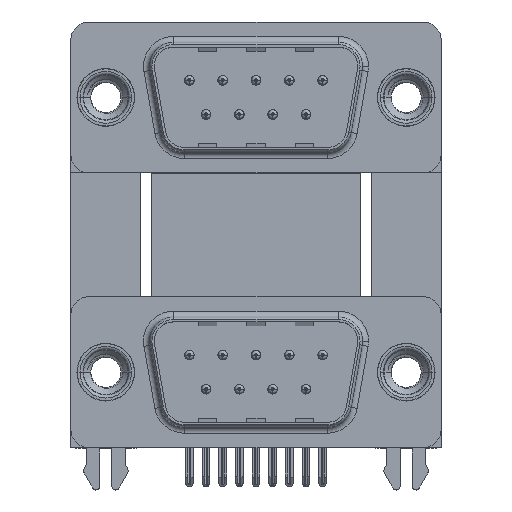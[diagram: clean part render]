
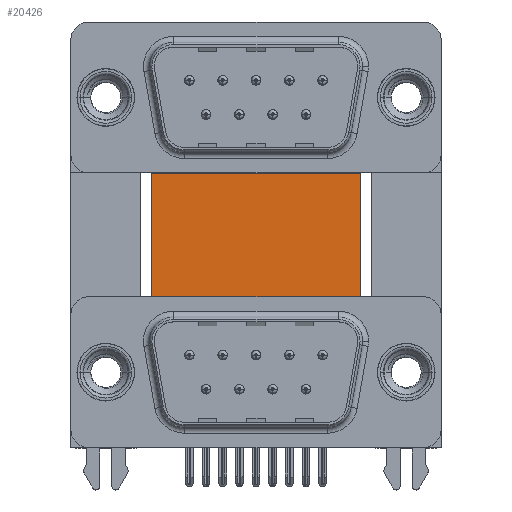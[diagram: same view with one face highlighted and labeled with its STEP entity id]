
A CAD part, top view. The second image highlights one B-rep face of the part: STEP entity #20426.
In plain terms, the highlighted planar face has unit normal (0, 0, 1).
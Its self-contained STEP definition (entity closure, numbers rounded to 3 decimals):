
#154 = VERTEX_POINT ( 'NONE', #6405 ) ;
#307 = CARTESIAN_POINT ( 'NONE',  ( 2.9, -4.635, -12. ) ) ;
#1339 = CARTESIAN_POINT ( 'NONE',  ( 2.9, -3.735, -12. ) ) ;
#1932 = CARTESIAN_POINT ( 'NONE',  ( 22.59, -4.635, -12. ) ) ;
#2231 = EDGE_CURVE ( 'NONE', #25039, #14786, #10625, .T. ) ;
#2434 = EDGE_CURVE ( 'NONE', #154, #4086, #5527, .T. ) ;
#2470 = LINE ( 'NONE', #21363, #23860 ) ;
#2626 = CARTESIAN_POINT ( 'NONE',  ( 21.2, -0.735, -12. ) ) ;
#2739 = LINE ( 'NONE', #11279, #12707 ) ;
#2900 = ORIENTED_EDGE ( 'NONE', *, *, #4448, .T. ) ;
#3172 = DIRECTION ( 'NONE',  ( 0., 0., -1. ) ) ;
#3363 = ORIENTED_EDGE ( 'NONE', *, *, #2231, .T. ) ;
#4086 = VERTEX_POINT ( 'NONE', #4702 ) ;
#4448 = EDGE_CURVE ( 'NONE', #24860, #20365, #23354, .T. ) ;
#4702 = CARTESIAN_POINT ( 'NONE',  ( 21.2, 16.585, -12. ) ) ;
#4965 = EDGE_CURVE ( 'NONE', #22693, #17643, #21934, .T. ) ;
#5283 = PLANE ( 'NONE',  #25709 ) ;
#5298 = CARTESIAN_POINT ( 'NONE',  ( 22.09, -4.635, -12. ) ) ;
#5527 = LINE ( 'NONE', #14062, #19161 ) ;
#6221 = CARTESIAN_POINT ( 'NONE',  ( 3.79, -0.735, -12. ) ) ;
#6405 = CARTESIAN_POINT ( 'NONE',  ( 3.79, 16.585, -12. ) ) ;
#6859 = EDGE_CURVE ( 'NONE', #14786, #15094, #2739, .T. ) ;
#7507 = CARTESIAN_POINT ( 'NONE',  ( 22.59, -4.635, -12. ) ) ;
#7637 = VECTOR ( 'NONE', #10480, 1000. ) ;
#8508 = CARTESIAN_POINT ( 'NONE',  ( 22.09, -3.735, -12. ) ) ;
#8879 = ORIENTED_EDGE ( 'NONE', *, *, #6859, .T. ) ;
#9047 = CARTESIAN_POINT ( 'NONE',  ( 2.9, -3.735, -12. ) ) ;
#9178 = DIRECTION ( 'NONE',  ( 1., 0., 0. ) ) ;
#9494 = DIRECTION ( 'NONE',  ( 1., 0., 0. ) ) ;
#9761 = FACE_OUTER_BOUND ( 'NONE', #24879, .T. ) ;
#10480 = DIRECTION ( 'NONE',  ( -0.336, 0.942, 0. ) ) ;
#10612 = CARTESIAN_POINT ( 'NONE',  ( 21.2, 16.585, -12. ) ) ;
#10625 = LINE ( 'NONE', #13127, #11577 ) ;
#10627 = VECTOR ( 'NONE', #19293, 1000. ) ;
#10759 = DIRECTION ( 'NONE',  ( -0.336, -0.942, 0. ) ) ;
#11019 = ORIENTED_EDGE ( 'NONE', *, *, #18317, .T. ) ;
#11279 = CARTESIAN_POINT ( 'NONE',  ( 2.9, -4.635, -12. ) ) ;
#11577 = VECTOR ( 'NONE', #10759, 1000. ) ;
#11973 = DIRECTION ( 'NONE',  ( 1., 0., 0. ) ) ;
#12065 = ORIENTED_EDGE ( 'NONE', *, *, #4965, .T. ) ;
#12707 = VECTOR ( 'NONE', #9178, 1000. ) ;
#12741 = EDGE_CURVE ( 'NONE', #20365, #22693, #24034, .T. ) ;
#13127 = CARTESIAN_POINT ( 'NONE',  ( 2.4, -4.635, -12. ) ) ;
#13813 = CARTESIAN_POINT ( 'NONE',  ( 3.79, 16.585, -12. ) ) ;
#14062 = CARTESIAN_POINT ( 'NONE',  ( 3.79, 16.585, -12. ) ) ;
#14197 = VECTOR ( 'NONE', #17036, 1000. ) ;
#14786 = VERTEX_POINT ( 'NONE', #15751 ) ;
#14810 = LINE ( 'NONE', #10612, #21773 ) ;
#15094 = VERTEX_POINT ( 'NONE', #307 ) ;
#15633 = LINE ( 'NONE', #9047, #23590 ) ;
#15751 = CARTESIAN_POINT ( 'NONE',  ( 2.4, -4.635, -12. ) ) ;
#15774 = CARTESIAN_POINT ( 'NONE',  ( 22.09, -3.735, -12. ) ) ;
#16980 = ORIENTED_EDGE ( 'NONE', *, *, #23608, .F. ) ;
#17036 = DIRECTION ( 'NONE',  ( 0., -1., 0. ) ) ;
#17361 = CARTESIAN_POINT ( 'NONE',  ( 3.79, -3.735, -12. ) ) ;
#17643 = VERTEX_POINT ( 'NONE', #7507 ) ;
#18317 = EDGE_CURVE ( 'NONE', #17643, #23633, #21104, .T. ) ;
#19161 = VECTOR ( 'NONE', #11973, 1000. ) ;
#19256 = DIRECTION ( 'NONE',  ( 0., -1., 0. ) ) ;
#19293 = DIRECTION ( 'NONE',  ( 1., 0., 0. ) ) ;
#20233 = EDGE_CURVE ( 'NONE', #154, #25039, #2470, .T. ) ;
#20288 = CARTESIAN_POINT ( 'NONE',  ( 22.09, -4.635, -12. ) ) ;
#20365 = VERTEX_POINT ( 'NONE', #15774 ) ;
#20426 = ADVANCED_FACE ( 'NONE', ( #9761 ), #5283, .F. ) ;
#21104 = LINE ( 'NONE', #1932, #7637 ) ;
#21363 = CARTESIAN_POINT ( 'NONE',  ( 3.79, 16.585, -12. ) ) ;
#21773 = VECTOR ( 'NONE', #23324, 1000. ) ;
#21934 = LINE ( 'NONE', #5298, #23141 ) ;
#22279 = ORIENTED_EDGE ( 'NONE', *, *, #2434, .F. ) ;
#22693 = VERTEX_POINT ( 'NONE', #20288 ) ;
#23141 = VECTOR ( 'NONE', #9494, 1000. ) ;
#23324 = DIRECTION ( 'NONE',  ( 0., -1., 0. ) ) ;
#23354 = LINE ( 'NONE', #17361, #10627 ) ;
#23590 = VECTOR ( 'NONE', #26408, 1000. ) ;
#23608 = EDGE_CURVE ( 'NONE', #4086, #23633, #14810, .T. ) ;
#23633 = VERTEX_POINT ( 'NONE', #2626 ) ;
#23860 = VECTOR ( 'NONE', #19256, 1000. ) ;
#24034 = LINE ( 'NONE', #8508, #14197 ) ;
#24581 = DIRECTION ( 'NONE',  ( -1., 0., 0. ) ) ;
#24717 = EDGE_CURVE ( 'NONE', #15094, #24860, #15633, .T. ) ;
#24860 = VERTEX_POINT ( 'NONE', #1339 ) ;
#24879 = EDGE_LOOP ( 'NONE', ( #2900, #27538, #12065, #11019, #16980, #22279, #25084, #3363, #8879, #27430 ) ) ;
#25039 = VERTEX_POINT ( 'NONE', #6221 ) ;
#25084 = ORIENTED_EDGE ( 'NONE', *, *, #20233, .T. ) ;
#25709 = AXIS2_PLACEMENT_3D ( 'NONE', #13813, #3172, #24581 ) ;
#26408 = DIRECTION ( 'NONE',  ( 0., 1., 0. ) ) ;
#27430 = ORIENTED_EDGE ( 'NONE', *, *, #24717, .T. ) ;
#27538 = ORIENTED_EDGE ( 'NONE', *, *, #12741, .T. ) ;
